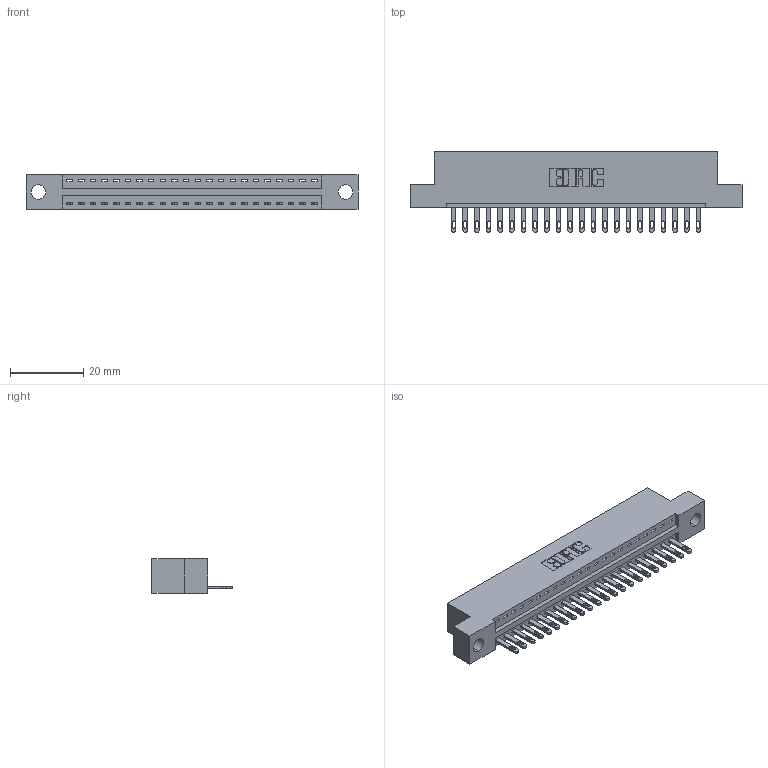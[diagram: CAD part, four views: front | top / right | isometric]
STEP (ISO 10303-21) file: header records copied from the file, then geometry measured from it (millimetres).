
FILE_DESCRIPTION (( 'STEP AP203' ), '1' );
FILE_NAME ('346-022-500-104.STEP', '2022-05-05T18:52:17', ( '' ), ( '' ), 'SwSTEP 2.0', 'SolidWorks 2020', '' );
FILE_SCHEMA (( 'CONFIG_CONTROL_DESIGN' ));
Length unit declared in the file: inch
Products named in the file (3): 346 Part_Flush Mounting Lugs - 0.156 Dia-TH; 346-022-500-104; 345-292-001_345-293-100
Assembly tree (23 placements, depth 2):
  346-022-500-104
    346 Part_Flush Mounting Lugs - 0.156 Dia-TH
    345-292-001_345-293-100  x22
Bounding box: 90.42 x 21.84 x 9.4 mm (x, y, z)
Volume: 8425.4 mm3; surface area: 10203.4 mm2
Topology: 23 solids, 23 shells, 1324 faces, 4061 edges, 2706 vertices
Faces by surface type: plane 838, cylinder 486
Entity records: 16695 total; most frequent: CARTESIAN_POINT 2876, ORIENTED_EDGE 2830, DIRECTION 2563, EDGE_CURVE 1415, VECTOR 1191, LINE 1191, VERTEX_POINT 942, AXIS2_PLACEMENT_3D 686
